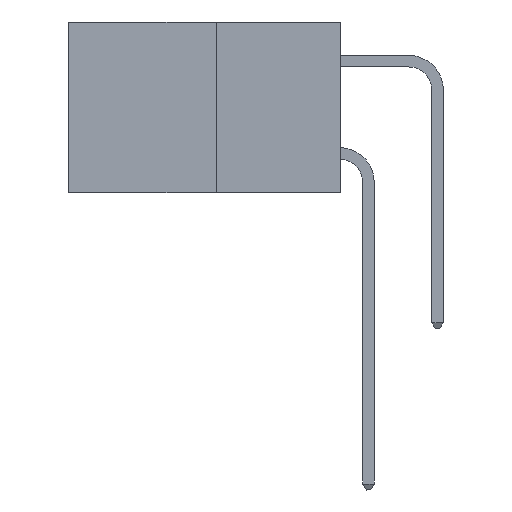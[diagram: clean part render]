
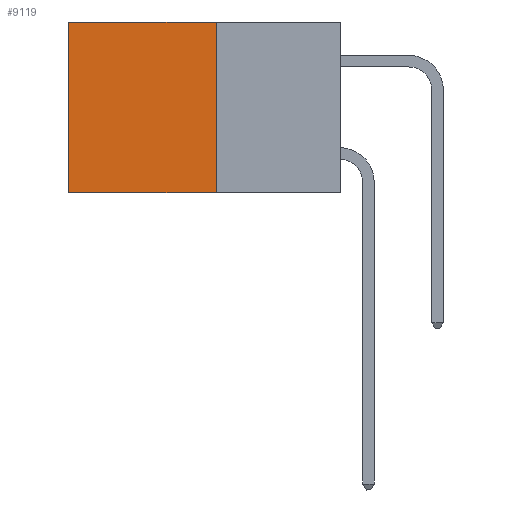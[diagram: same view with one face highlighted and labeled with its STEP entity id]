
A CAD part, left-side view. The second image highlights one B-rep face of the part: STEP entity #9119.
In plain terms, the highlighted planar face has unit normal (-1, 0, 0).
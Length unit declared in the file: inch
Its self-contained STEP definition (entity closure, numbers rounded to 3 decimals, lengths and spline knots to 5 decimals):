
#296 = ORIENTED_EDGE ( 'NONE', *, *, #13169, .F. ) ;
#803 = PLANE ( 'NONE',  #2392 ) ;
#828 = VERTEX_POINT ( 'NONE', #4499 ) ;
#1025 = CARTESIAN_POINT ( 'NONE',  ( 0.277, 0.59, 0. ) ) ;
#2125 = ORIENTED_EDGE ( 'NONE', *, *, #13911, .F. ) ;
#2198 = CARTESIAN_POINT ( 'NONE',  ( 0.277, 0.27, 0. ) ) ;
#2392 = AXIS2_PLACEMENT_3D ( 'NONE', #15626, #3756, #14210 ) ;
#2893 = VECTOR ( 'NONE', #15838, 39.37008 ) ;
#3087 = LINE ( 'NONE', #4479, #11074 ) ;
#3756 = DIRECTION ( 'NONE',  ( 1., 0., 0. ) ) ;
#4479 = CARTESIAN_POINT ( 'NONE',  ( 0.277, 0.59, -0.37 ) ) ;
#4499 = CARTESIAN_POINT ( 'NONE',  ( 0.277, 0.59, -0.37 ) ) ;
#5130 = EDGE_CURVE ( 'NONE', #14989, #13930, #13738, .T. ) ;
#5577 = CARTESIAN_POINT ( 'NONE',  ( 0.277, 0.27, -0.37 ) ) ;
#5947 = DIRECTION ( 'NONE',  ( 0., 0., -1. ) ) ;
#6953 = CARTESIAN_POINT ( 'NONE',  ( 0.277, 0.27, -0.37 ) ) ;
#7389 = LINE ( 'NONE', #10282, #18621 ) ;
#7623 = ORIENTED_EDGE ( 'NONE', *, *, #8798, .T. ) ;
#7965 = VERTEX_POINT ( 'NONE', #5577 ) ;
#8798 = EDGE_CURVE ( 'NONE', #13930, #828, #3087, .T. ) ;
#9119 = ADVANCED_FACE ( 'NONE', ( #9437 ), #803, .F. ) ;
#9338 = VECTOR ( 'NONE', #12647, 39.37008 ) ;
#9437 = FACE_OUTER_BOUND ( 'NONE', #14617, .T. ) ;
#9751 = ORIENTED_EDGE ( 'NONE', *, *, #5130, .T. ) ;
#10282 = CARTESIAN_POINT ( 'NONE',  ( 0.277, 0.27, -0.37 ) ) ;
#11074 = VECTOR ( 'NONE', #5947, 39.37008 ) ;
#11763 = DIRECTION ( 'NONE',  ( 0., 1., 0. ) ) ;
#12647 = DIRECTION ( 'NONE',  ( 0., 1., 0. ) ) ;
#13169 = EDGE_CURVE ( 'NONE', #7965, #828, #7389, .T. ) ;
#13738 = LINE ( 'NONE', #2198, #9338 ) ;
#13911 = EDGE_CURVE ( 'NONE', #14989, #7965, #17703, .T. ) ;
#13930 = VERTEX_POINT ( 'NONE', #1025 ) ;
#14021 = CARTESIAN_POINT ( 'NONE',  ( 0.277, 0.27, 0. ) ) ;
#14210 = DIRECTION ( 'NONE',  ( 0., 0., -1. ) ) ;
#14617 = EDGE_LOOP ( 'NONE', ( #7623, #296, #2125, #9751 ) ) ;
#14989 = VERTEX_POINT ( 'NONE', #14021 ) ;
#15626 = CARTESIAN_POINT ( 'NONE',  ( 0.277, 0.27, -0.37 ) ) ;
#15838 = DIRECTION ( 'NONE',  ( 0., 0., -1. ) ) ;
#17703 = LINE ( 'NONE', #6953, #2893 ) ;
#18621 = VECTOR ( 'NONE', #11763, 39.37008 ) ;
